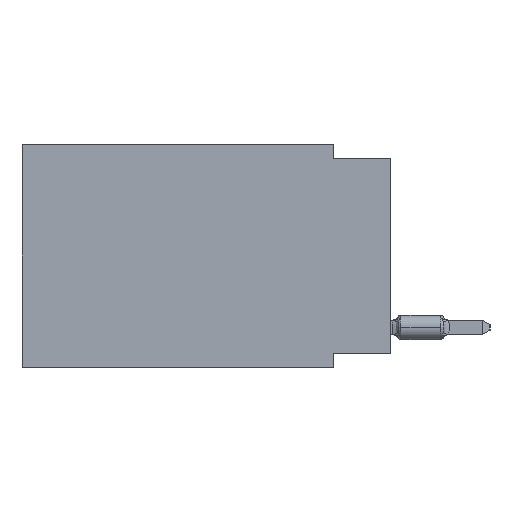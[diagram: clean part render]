
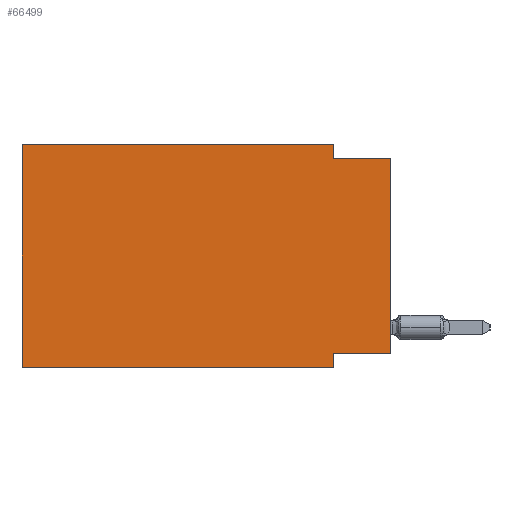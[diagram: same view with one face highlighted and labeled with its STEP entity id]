
A CAD part, left-side view. The second image highlights one B-rep face of the part: STEP entity #66499.
In plain terms, the highlighted planar face has unit normal (-1, 0, 0).
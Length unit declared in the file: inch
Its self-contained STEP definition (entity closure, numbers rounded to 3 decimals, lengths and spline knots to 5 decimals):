
#409 = VECTOR ( 'NONE', #45794, 39.37008 ) ;
#1392 = CARTESIAN_POINT ( 'NONE',  ( 0., 0., -0.025 ) ) ;
#3590 = CARTESIAN_POINT ( 'NONE',  ( 0., 0., -0.365 ) ) ;
#4060 = VERTEX_POINT ( 'NONE', #1392 ) ;
#4872 = VECTOR ( 'NONE', #28232, 39.37008 ) ;
#5642 = CARTESIAN_POINT ( 'NONE',  ( 0., 0.645, -0.39 ) ) ;
#5726 = EDGE_CURVE ( 'NONE', #47112, #4060, #42087, .T. ) ;
#6021 = VECTOR ( 'NONE', #6849, 39.37008 ) ;
#6849 = DIRECTION ( 'NONE',  ( 0., 0., 1. ) ) ;
#7807 = CARTESIAN_POINT ( 'NONE',  ( 0., 0.1, 0. ) ) ;
#7918 = VERTEX_POINT ( 'NONE', #19216 ) ;
#11333 = LINE ( 'NONE', #23150, #42885 ) ;
#11719 = LINE ( 'NONE', #62649, #44753 ) ;
#12987 = ORIENTED_EDGE ( 'NONE', *, *, #25244, .F. ) ;
#13896 = ORIENTED_EDGE ( 'NONE', *, *, #14314, .F. ) ;
#14314 = EDGE_CURVE ( 'NONE', #28704, #4060, #14678, .T. ) ;
#14678 = LINE ( 'NONE', #35502, #409 ) ;
#15325 = CARTESIAN_POINT ( 'NONE',  ( 0., 0.1, -0.39 ) ) ;
#16344 = LINE ( 'NONE', #15325, #46763 ) ;
#18073 = DIRECTION ( 'NONE',  ( 0., -1., 0. ) ) ;
#19076 = CARTESIAN_POINT ( 'NONE',  ( 0., 0.645, -0.39 ) ) ;
#19216 = CARTESIAN_POINT ( 'NONE',  ( 0., 0.645, 0. ) ) ;
#20574 = AXIS2_PLACEMENT_3D ( 'NONE', #67005, #50275, #34512 ) ;
#21582 = DIRECTION ( 'NONE',  ( 0., 0., -1. ) ) ;
#22561 = CARTESIAN_POINT ( 'NONE',  ( 0., 0., 0. ) ) ;
#23150 = CARTESIAN_POINT ( 'NONE',  ( 0., 0.1, 0. ) ) ;
#24195 = LINE ( 'NONE', #19076, #44048 ) ;
#25244 = EDGE_CURVE ( 'NONE', #45107, #28704, #11333, .T. ) ;
#26296 = VECTOR ( 'NONE', #18073, 39.37008 ) ;
#28232 = DIRECTION ( 'NONE',  ( 0., 1., 0. ) ) ;
#28336 = CARTESIAN_POINT ( 'NONE',  ( 0., 0.645, 0. ) ) ;
#28688 = ORIENTED_EDGE ( 'NONE', *, *, #5726, .T. ) ;
#28704 = VERTEX_POINT ( 'NONE', #40200 ) ;
#29406 = FACE_OUTER_BOUND ( 'NONE', #37961, .T. ) ;
#31726 = DIRECTION ( 'NONE',  ( 0., 0., -1. ) ) ;
#33342 = CARTESIAN_POINT ( 'NONE',  ( 0., 0., -0.365 ) ) ;
#33345 = EDGE_CURVE ( 'NONE', #35060, #62887, #16344, .T. ) ;
#34512 = DIRECTION ( 'NONE',  ( 0., 0., -1. ) ) ;
#35060 = VERTEX_POINT ( 'NONE', #45319 ) ;
#35502 = CARTESIAN_POINT ( 'NONE',  ( 0., 0., -0.025 ) ) ;
#36336 = EDGE_CURVE ( 'NONE', #7918, #45107, #59773, .T. ) ;
#37961 = EDGE_LOOP ( 'NONE', ( #28688, #13896, #12987, #39523, #52037, #45042, #56055, #58113 ) ) ;
#39523 = ORIENTED_EDGE ( 'NONE', *, *, #36336, .F. ) ;
#39918 = DIRECTION ( 'NONE',  ( 0., -1., 0. ) ) ;
#40200 = CARTESIAN_POINT ( 'NONE',  ( 0., 0.1, -0.025 ) ) ;
#41882 = VERTEX_POINT ( 'NONE', #5642 ) ;
#42087 = LINE ( 'NONE', #22561, #6021 ) ;
#42885 = VECTOR ( 'NONE', #21582, 39.37008 ) ;
#43395 = EDGE_CURVE ( 'NONE', #41882, #7918, #11719, .T. ) ;
#43639 = LINE ( 'NONE', #33342, #4872 ) ;
#44048 = VECTOR ( 'NONE', #39918, 39.37008 ) ;
#44753 = VECTOR ( 'NONE', #63331, 39.37008 ) ;
#45042 = ORIENTED_EDGE ( 'NONE', *, *, #50865, .T. ) ;
#45107 = VERTEX_POINT ( 'NONE', #7807 ) ;
#45319 = CARTESIAN_POINT ( 'NONE',  ( 0., 0.1, -0.365 ) ) ;
#45794 = DIRECTION ( 'NONE',  ( 0., -1., 0. ) ) ;
#46763 = VECTOR ( 'NONE', #31726, 39.37008 ) ;
#47112 = VERTEX_POINT ( 'NONE', #3590 ) ;
#50275 = DIRECTION ( 'NONE',  ( 1., 0., 0. ) ) ;
#50666 = CARTESIAN_POINT ( 'NONE',  ( 0., 0.1, -0.39 ) ) ;
#50865 = EDGE_CURVE ( 'NONE', #41882, #62887, #24195, .T. ) ;
#50943 = PLANE ( 'NONE',  #20574 ) ;
#51632 = EDGE_CURVE ( 'NONE', #47112, #35060, #43639, .T. ) ;
#52037 = ORIENTED_EDGE ( 'NONE', *, *, #43395, .F. ) ;
#56055 = ORIENTED_EDGE ( 'NONE', *, *, #33345, .F. ) ;
#58113 = ORIENTED_EDGE ( 'NONE', *, *, #51632, .F. ) ;
#59773 = LINE ( 'NONE', #28336, #26296 ) ;
#62649 = CARTESIAN_POINT ( 'NONE',  ( 0., 0.645, 0. ) ) ;
#62887 = VERTEX_POINT ( 'NONE', #50666 ) ;
#63331 = DIRECTION ( 'NONE',  ( 0., 0., 1. ) ) ;
#66499 = ADVANCED_FACE ( 'NONE', ( #29406 ), #50943, .F. ) ;
#67005 = CARTESIAN_POINT ( 'NONE',  ( 0., 0.645, 0. ) ) ;
